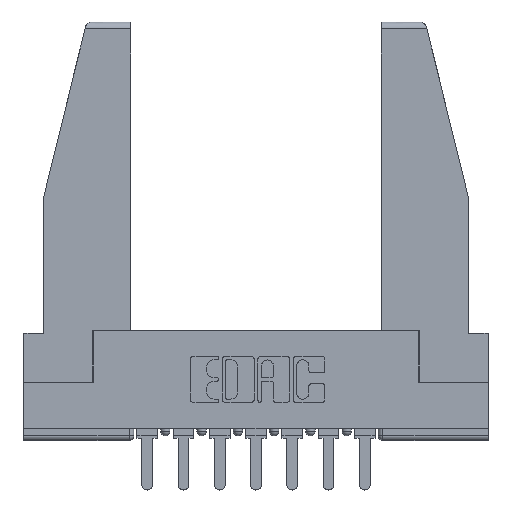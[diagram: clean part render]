
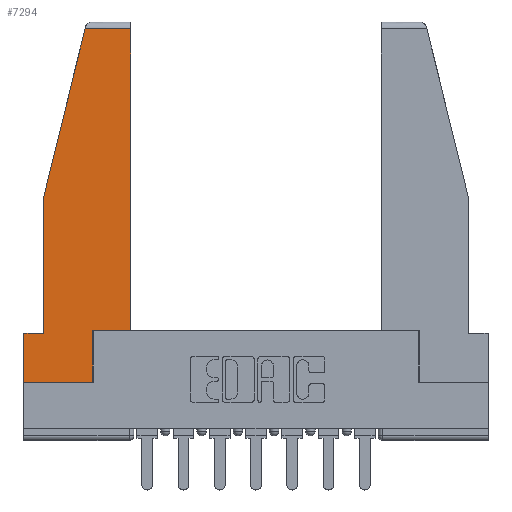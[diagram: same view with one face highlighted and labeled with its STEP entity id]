
A CAD part, top view. The second image highlights one B-rep face of the part: STEP entity #7294.
In plain terms, the highlighted planar face has unit normal (0, 0, 1).
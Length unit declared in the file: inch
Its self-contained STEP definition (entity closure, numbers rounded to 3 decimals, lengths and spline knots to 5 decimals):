
#38 = ORIENTED_EDGE ( 'NONE', *, *, #2766, .T. ) ;
#60 = EDGE_CURVE ( 'NONE', #1233, #9650, #3915, .T. ) ;
#203 = DIRECTION ( 'NONE',  ( 1., 0., 0. ) ) ;
#828 = CARTESIAN_POINT ( 'NONE',  ( 0., 1.52, 0. ) ) ;
#839 = ORIENTED_EDGE ( 'NONE', *, *, #7245, .T. ) ;
#849 = CARTESIAN_POINT ( 'NONE',  ( 0., 0.21, 0. ) ) ;
#1035 = DIRECTION ( 'NONE',  ( -1., 0., 0. ) ) ;
#1144 = VERTEX_POINT ( 'NONE', #2170 ) ;
#1233 = VERTEX_POINT ( 'NONE', #5709 ) ;
#1503 = DIRECTION ( 'NONE',  ( 1., 0., 0. ) ) ;
#1521 = CARTESIAN_POINT ( 'NONE',  ( 0., 0.21, 0. ) ) ;
#1840 = EDGE_CURVE ( 'NONE', #11783, #9652, #13369, .T. ) ;
#1887 = VECTOR ( 'NONE', #8658, 39.37008 ) ;
#2130 = DIRECTION ( 'NONE',  ( 0., 1., 0. ) ) ;
#2170 = CARTESIAN_POINT ( 'NONE',  ( 0.297, 0.223, 0. ) ) ;
#2179 = VECTOR ( 'NONE', #2130, 39.37008 ) ;
#2507 = ORIENTED_EDGE ( 'NONE', *, *, #60, .T. ) ;
#2609 = VECTOR ( 'NONE', #1503, 39.37008 ) ;
#2766 = EDGE_CURVE ( 'NONE', #8760, #1233, #5363, .T. ) ;
#2950 = EDGE_CURVE ( 'NONE', #9652, #11543, #7801, .T. ) ;
#3225 = LINE ( 'NONE', #4384, #2179 ) ;
#3438 = CARTESIAN_POINT ( 'NONE',  ( 0.086, 0.8, 0. ) ) ;
#3693 = CARTESIAN_POINT ( 'NONE',  ( 0., 0., 0. ) ) ;
#3884 = VECTOR ( 'NONE', #1035, 39.37008 ) ;
#3891 = ORIENTED_EDGE ( 'NONE', *, *, #7317, .T. ) ;
#3915 = LINE ( 'NONE', #828, #3884 ) ;
#4192 = LINE ( 'NONE', #12503, #11680 ) ;
#4384 = CARTESIAN_POINT ( 'NONE',  ( 0.297, 0., 0. ) ) ;
#4395 = LINE ( 'NONE', #3438, #6256 ) ;
#4403 = ORIENTED_EDGE ( 'NONE', *, *, #1840, .T. ) ;
#4523 = AXIS2_PLACEMENT_3D ( 'NONE', #4670, #6713, #203 ) ;
#4670 = CARTESIAN_POINT ( 'NONE',  ( 0., 0., 0. ) ) ;
#5069 = DIRECTION ( 'NONE',  ( -1., 0., 0. ) ) ;
#5077 = CARTESIAN_POINT ( 'NONE',  ( 0., 0., 0. ) ) ;
#5363 = LINE ( 'NONE', #9390, #6205 ) ;
#5577 = LINE ( 'NONE', #10746, #1887 ) ;
#5709 = CARTESIAN_POINT ( 'NONE',  ( 0.461, 1.52, 0. ) ) ;
#6094 = CARTESIAN_POINT ( 'NONE',  ( 0., 0.21, 0. ) ) ;
#6205 = VECTOR ( 'NONE', #6325, 39.37008 ) ;
#6256 = VECTOR ( 'NONE', #8827, 39.37008 ) ;
#6325 = DIRECTION ( 'NONE',  ( 0., 1., 0. ) ) ;
#6513 = CARTESIAN_POINT ( 'NONE',  ( 0.086, 0.8, 0. ) ) ;
#6713 = DIRECTION ( 'NONE',  ( 0., 0., 1. ) ) ;
#6997 = EDGE_CURVE ( 'NONE', #1144, #8760, #5577, .T. ) ;
#7245 = EDGE_CURVE ( 'NONE', #9650, #7357, #4192, .T. ) ;
#7294 = ADVANCED_FACE ( 'NONE', ( #9708 ), #12840, .T. ) ;
#7317 = EDGE_CURVE ( 'NONE', #7357, #11783, #4395, .T. ) ;
#7357 = VERTEX_POINT ( 'NONE', #6513 ) ;
#7452 = ORIENTED_EDGE ( 'NONE', *, *, #2950, .T. ) ;
#7569 = VERTEX_POINT ( 'NONE', #11249 ) ;
#7801 = LINE ( 'NONE', #1521, #11620 ) ;
#8218 = EDGE_LOOP ( 'NONE', ( #38, #2507, #839, #3891, #4403, #7452, #9569, #9919, #11136 ) ) ;
#8240 = VECTOR ( 'NONE', #5069, 39.37008 ) ;
#8658 = DIRECTION ( 'NONE',  ( 1., 0., 0. ) ) ;
#8708 = DIRECTION ( 'NONE',  ( 0., -1., 0. ) ) ;
#8720 = CARTESIAN_POINT ( 'NONE',  ( 0.461, 0.223, 0. ) ) ;
#8760 = VERTEX_POINT ( 'NONE', #8720 ) ;
#8827 = DIRECTION ( 'NONE',  ( 0., -1., 0. ) ) ;
#9390 = CARTESIAN_POINT ( 'NONE',  ( 0.461, 0.223, 0. ) ) ;
#9569 = ORIENTED_EDGE ( 'NONE', *, *, #10835, .T. ) ;
#9650 = VERTEX_POINT ( 'NONE', #10205 ) ;
#9652 = VERTEX_POINT ( 'NONE', #849 ) ;
#9708 = FACE_OUTER_BOUND ( 'NONE', #8218, .T. ) ;
#9828 = LINE ( 'NONE', #3693, #2609 ) ;
#9919 = ORIENTED_EDGE ( 'NONE', *, *, #11673, .T. ) ;
#10205 = CARTESIAN_POINT ( 'NONE',  ( 0.2636, 1.52, 0. ) ) ;
#10379 = DIRECTION ( 'NONE',  ( -0.239, -0.971, 0. ) ) ;
#10746 = CARTESIAN_POINT ( 'NONE',  ( 0.297, 0.223, 0. ) ) ;
#10835 = EDGE_CURVE ( 'NONE', #11543, #7569, #9828, .T. ) ;
#11136 = ORIENTED_EDGE ( 'NONE', *, *, #6997, .T. ) ;
#11249 = CARTESIAN_POINT ( 'NONE',  ( 0.297, 0., 0. ) ) ;
#11543 = VERTEX_POINT ( 'NONE', #5077 ) ;
#11620 = VECTOR ( 'NONE', #8708, 39.37008 ) ;
#11673 = EDGE_CURVE ( 'NONE', #7569, #1144, #3225, .T. ) ;
#11680 = VECTOR ( 'NONE', #10379, 39.37008 ) ;
#11783 = VERTEX_POINT ( 'NONE', #12896 ) ;
#12503 = CARTESIAN_POINT ( 'NONE',  ( 0.271, 1.55, 0. ) ) ;
#12840 = PLANE ( 'NONE',  #4523 ) ;
#12896 = CARTESIAN_POINT ( 'NONE',  ( 0.086, 0.21, 0. ) ) ;
#13369 = LINE ( 'NONE', #6094, #8240 ) ;
